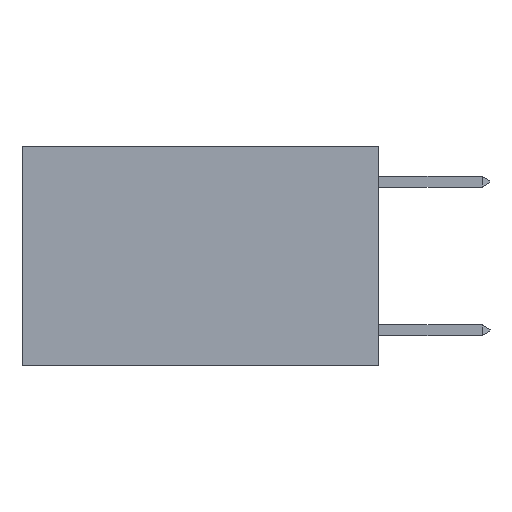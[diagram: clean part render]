
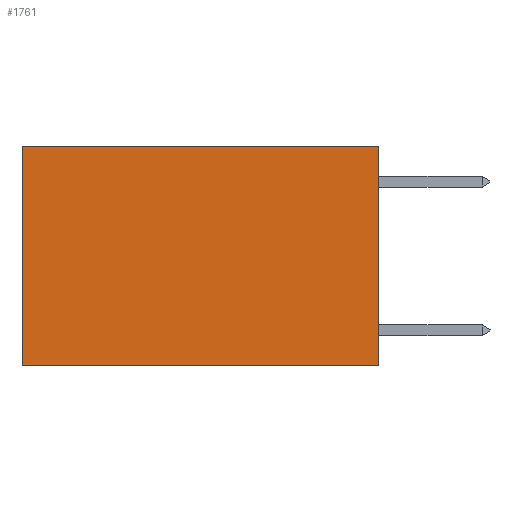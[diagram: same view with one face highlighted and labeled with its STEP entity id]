
A CAD part, left-side view. The second image highlights one B-rep face of the part: STEP entity #1761.
In plain terms, the highlighted planar face has unit normal (-1, 0, 0).
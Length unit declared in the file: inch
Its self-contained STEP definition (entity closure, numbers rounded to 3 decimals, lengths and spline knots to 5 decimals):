
#493 = VERTEX_POINT ( 'NONE', #18356 ) ;
#1186 = CARTESIAN_POINT ( 'NONE',  ( 0.2625, 0.6, -0.37 ) ) ;
#1761 = ADVANCED_FACE ( 'NONE', ( #2246 ), #16570, .F. ) ;
#2246 = FACE_OUTER_BOUND ( 'NONE', #4636, .T. ) ;
#2963 = LINE ( 'NONE', #9774, #3473 ) ;
#3100 = CARTESIAN_POINT ( 'NONE',  ( 0.2625, 0.6, 0. ) ) ;
#3329 = ORIENTED_EDGE ( 'NONE', *, *, #22230, .T. ) ;
#3455 = EDGE_CURVE ( 'NONE', #493, #9505, #2963, .T. ) ;
#3473 = VECTOR ( 'NONE', #9703, 39.37008 ) ;
#4636 = EDGE_LOOP ( 'NONE', ( #3329, #17361, #17746, #19147 ) ) ;
#4925 = DIRECTION ( 'NONE',  ( 0., 0., -1. ) ) ;
#5755 = CARTESIAN_POINT ( 'NONE',  ( 0.2625, 0.6, 0. ) ) ;
#6432 = CARTESIAN_POINT ( 'NONE',  ( 0.2625, 0., -0.37 ) ) ;
#7195 = VERTEX_POINT ( 'NONE', #1186 ) ;
#7957 = VECTOR ( 'NONE', #22840, 39.37008 ) ;
#8412 = LINE ( 'NONE', #3100, #17300 ) ;
#8435 = LINE ( 'NONE', #17706, #13140 ) ;
#8754 = LINE ( 'NONE', #21096, #7957 ) ;
#8858 = DIRECTION ( 'NONE',  ( 0., 1., 0. ) ) ;
#9505 = VERTEX_POINT ( 'NONE', #6432 ) ;
#9703 = DIRECTION ( 'NONE',  ( 0., 0., -1. ) ) ;
#9774 = CARTESIAN_POINT ( 'NONE',  ( 0.2625, 0., 0. ) ) ;
#10314 = AXIS2_PLACEMENT_3D ( 'NONE', #16597, #16098, #16204 ) ;
#11242 = VERTEX_POINT ( 'NONE', #5755 ) ;
#13140 = VECTOR ( 'NONE', #8858, 39.37008 ) ;
#16019 = EDGE_CURVE ( 'NONE', #493, #11242, #8754, .T. ) ;
#16098 = DIRECTION ( 'NONE',  ( 1., 0., 0. ) ) ;
#16204 = DIRECTION ( 'NONE',  ( 0., 0., -1. ) ) ;
#16570 = PLANE ( 'NONE',  #10314 ) ;
#16597 = CARTESIAN_POINT ( 'NONE',  ( 0.2625, 0., 0. ) ) ;
#17300 = VECTOR ( 'NONE', #4925, 39.37008 ) ;
#17361 = ORIENTED_EDGE ( 'NONE', *, *, #21786, .F. ) ;
#17706 = CARTESIAN_POINT ( 'NONE',  ( 0.2625, 0., -0.37 ) ) ;
#17746 = ORIENTED_EDGE ( 'NONE', *, *, #3455, .F. ) ;
#18356 = CARTESIAN_POINT ( 'NONE',  ( 0.2625, 0., 0. ) ) ;
#19147 = ORIENTED_EDGE ( 'NONE', *, *, #16019, .T. ) ;
#21096 = CARTESIAN_POINT ( 'NONE',  ( 0.2625, 0., 0. ) ) ;
#21786 = EDGE_CURVE ( 'NONE', #9505, #7195, #8435, .T. ) ;
#22230 = EDGE_CURVE ( 'NONE', #11242, #7195, #8412, .T. ) ;
#22840 = DIRECTION ( 'NONE',  ( 0., 1., 0. ) ) ;
